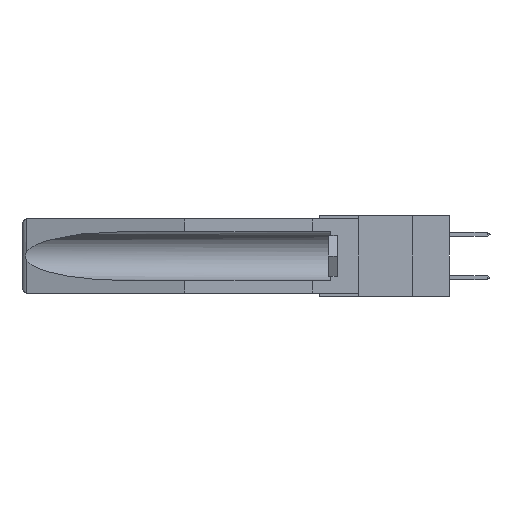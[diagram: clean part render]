
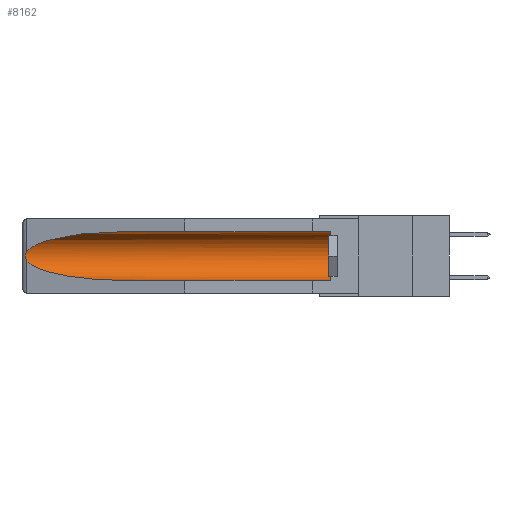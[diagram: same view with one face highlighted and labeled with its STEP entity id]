
A CAD part, left-side view. The second image highlights one B-rep face of the part: STEP entity #8162.
In plain terms, the highlighted cylindrical face has radius 2.857 mm (diameter 5.715 mm), a partial arc.
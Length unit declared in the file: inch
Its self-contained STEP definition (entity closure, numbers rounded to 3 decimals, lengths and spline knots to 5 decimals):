
#555 = VECTOR ( 'NONE', #12696, 39.37008 ) ;
#910 = CARTESIAN_POINT ( 'NONE',  ( 0.155, 1.07973, -0.284 ) ) ;
#1024 = VECTOR ( 'NONE', #14429, 39.37008 ) ;
#1299 = EDGE_CURVE ( 'NONE', #15900, #14493, #5994, .T. ) ;
#1452 = VERTEX_POINT ( 'NONE', #12951 ) ;
#2214 = CARTESIAN_POINT ( 'NONE',  ( 0.26537, 1.52718, -0.14972 ) ) ;
#2386 = CARTESIAN_POINT ( 'NONE',  ( 0.2673, 1.5327, -0.16383 ) ) ;
#2564 = CARTESIAN_POINT ( 'NONE',  ( 0.155, 0.126, -0.059 ) ) ;
#2850 = VERTEX_POINT ( 'NONE', #5811 ) ;
#3237 = DIRECTION ( 'NONE',  ( 0., 0., 1. ) ) ;
#3287 = EDGE_CURVE ( 'NONE', #2850, #8232, #20196, .T. ) ;
#3834 = ORIENTED_EDGE ( 'NONE', *, *, #9680, .T. ) ;
#3977 = ORIENTED_EDGE ( 'NONE', *, *, #14534, .F. ) ;
#4565 = CARTESIAN_POINT ( 'NONE',  ( 0.26654, 1.53092, -0.15636 ) ) ;
#4704 = CARTESIAN_POINT ( 'NONE',  ( 0.155, 1.07973, -0.059 ) ) ;
#5650 = CARTESIAN_POINT ( 'NONE',  ( 0.21114, 1.30732, -0.284 ) ) ;
#5811 = CARTESIAN_POINT ( 'NONE',  ( 0.26537, 1.52718, -0.19328 ) ) ;
#5994 = LINE ( 'NONE', #8439, #1024 ) ;
#6004 = EDGE_CURVE ( 'NONE', #17709, #2850, #11526, .T. ) ;
#6286 = CARTESIAN_POINT ( 'NONE',  ( 0.2673, 1.53269, -0.17917 ) ) ;
#6362 = CARTESIAN_POINT ( 'NONE',  ( 0.2675, 1.53308, -0.16763 ) ) ;
#7145 = CARTESIAN_POINT ( 'NONE',  ( 0.155, 0.126, -0.1715 ) ) ;
#7368 = CARTESIAN_POINT ( 'NONE',  ( 0.155, 1.07973, -0.284 ) ) ;
#7582 = CYLINDRICAL_SURFACE ( 'NONE', #18988, 0.1125 ) ;
#7622 = CARTESIAN_POINT ( 'NONE',  ( 0.26537, 1.52718, -0.14972 ) ) ;
#8096 = CARTESIAN_POINT ( 'NONE',  ( 0.26537, 1.52718, -0.19328 ) ) ;
#8162 = ADVANCED_FACE ( 'NONE', ( #19966 ), #7582, .F. ) ;
#8232 = VERTEX_POINT ( 'NONE', #910 ) ;
#8439 = CARTESIAN_POINT ( 'NONE',  ( 0.155, -0.30754, -0.059 ) ) ;
#9455 = ORIENTED_EDGE ( 'NONE', *, *, #14678, .T. ) ;
#9680 = EDGE_CURVE ( 'NONE', #14493, #17709, #13407, .T. ) ;
#10010 = CARTESIAN_POINT ( 'NONE',  ( 0.25451, 1.48313, -0.09465 ) ) ;
#10364 = ORIENTED_EDGE ( 'NONE', *, *, #6004, .T. ) ;
#11025 = CARTESIAN_POINT ( 'NONE',  ( 0.155, -0.30754, -0.1715 ) ) ;
#11526 = B_SPLINE_CURVE_WITH_KNOTS ( 'NONE', 3,
 ( #16425, #18229, #4565, #2386, #6362, #14098, #6286, #12111, #19952, #8096 ),
 .UNSPECIFIED., .F., .F.,
 ( 4, 2, 2, 2, 4 ),
 ( 0., 0.00029, 0.00058, 0.00087, 0.00117 ),
 .UNSPECIFIED. ) ;
#12111 = CARTESIAN_POINT ( 'NONE',  ( 0.26655, 1.53094, -0.18657 ) ) ;
#12306 = ORIENTED_EDGE ( 'NONE', *, *, #3287, .T. ) ;
#12696 = DIRECTION ( 'NONE',  ( 0., 1., 0. ) ) ;
#12951 = CARTESIAN_POINT ( 'NONE',  ( 0.155, 0.126, -0.284 ) ) ;
#13407 =( BOUNDED_CURVE ( )  B_SPLINE_CURVE ( 3, ( #19690, #13820, #10010, #2214 ),
 .UNSPECIFIED., .F., .F. ) 
 B_SPLINE_CURVE_WITH_KNOTS ( ( 4, 4 ),
 ( 4.71239, 6.08839 ),
 .UNSPECIFIED. ) 
 CURVE ( )  GEOMETRIC_REPRESENTATION_ITEM ( )  RATIONAL_B_SPLINE_CURVE ( ( 1., 0.848, 0.848, 1. ) ) 
 REPRESENTATION_ITEM ( '' )  );
#13523 = CARTESIAN_POINT ( 'NONE',  ( 0.25451, 1.48313, -0.24835 ) ) ;
#13820 = CARTESIAN_POINT ( 'NONE',  ( 0.21114, 1.30732, -0.059 ) ) ;
#14098 = CARTESIAN_POINT ( 'NONE',  ( 0.2675, 1.53308, -0.17534 ) ) ;
#14429 = DIRECTION ( 'NONE',  ( 0., 1., 0. ) ) ;
#14493 = VERTEX_POINT ( 'NONE', #4704 ) ;
#14534 = EDGE_CURVE ( 'NONE', #1452, #8232, #17297, .T. ) ;
#14606 = AXIS2_PLACEMENT_3D ( 'NONE', #7145, #18992, #17098 ) ;
#14678 = EDGE_CURVE ( 'NONE', #1452, #15900, #20043, .T. ) ;
#14779 = CARTESIAN_POINT ( 'NONE',  ( 0.155, -0.30754, -0.284 ) ) ;
#15099 = DIRECTION ( 'NONE',  ( 0., 1., 0. ) ) ;
#15900 = VERTEX_POINT ( 'NONE', #2564 ) ;
#16425 = CARTESIAN_POINT ( 'NONE',  ( 0.26537, 1.52718, -0.14972 ) ) ;
#17098 = DIRECTION ( 'NONE',  ( 0., 0., 1. ) ) ;
#17239 = CARTESIAN_POINT ( 'NONE',  ( 0.26537, 1.52718, -0.19328 ) ) ;
#17297 = LINE ( 'NONE', #14779, #555 ) ;
#17709 = VERTEX_POINT ( 'NONE', #7622 ) ;
#18229 = CARTESIAN_POINT ( 'NONE',  ( 0.26597, 1.52961, -0.15275 ) ) ;
#18988 = AXIS2_PLACEMENT_3D ( 'NONE', #11025, #15099, #3237 ) ;
#18992 = DIRECTION ( 'NONE',  ( 0., -1., 0. ) ) ;
#19690 = CARTESIAN_POINT ( 'NONE',  ( 0.155, 1.07973, -0.059 ) ) ;
#19952 = CARTESIAN_POINT ( 'NONE',  ( 0.26597, 1.5296, -0.19026 ) ) ;
#19966 = FACE_OUTER_BOUND ( 'NONE', #24881, .T. ) ;
#20043 = CIRCLE ( 'NONE', #14606, 0.1125 ) ;
#20196 =( BOUNDED_CURVE ( )  B_SPLINE_CURVE ( 3, ( #17239, #13523, #5650, #7368 ),
 .UNSPECIFIED., .F., .F. ) 
 B_SPLINE_CURVE_WITH_KNOTS ( ( 4, 4 ),
 ( 0.1948, 1.5708 ),
 .UNSPECIFIED. ) 
 CURVE ( )  GEOMETRIC_REPRESENTATION_ITEM ( )  RATIONAL_B_SPLINE_CURVE ( ( 1., 0.848, 0.848, 1. ) ) 
 REPRESENTATION_ITEM ( '' )  );
#24196 = ORIENTED_EDGE ( 'NONE', *, *, #1299, .T. ) ;
#24881 = EDGE_LOOP ( 'NONE', ( #3834, #10364, #12306, #3977, #9455, #24196 ) ) ;
